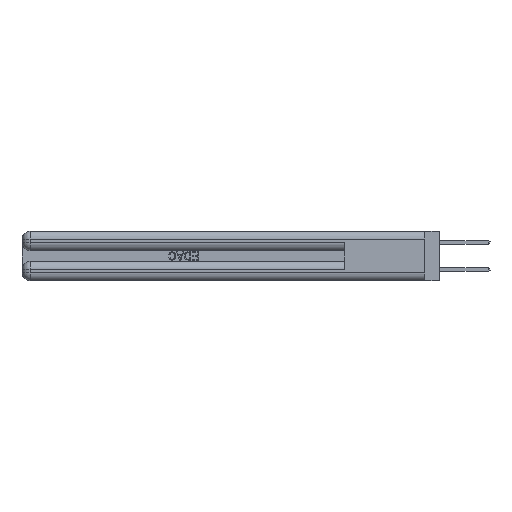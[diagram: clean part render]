
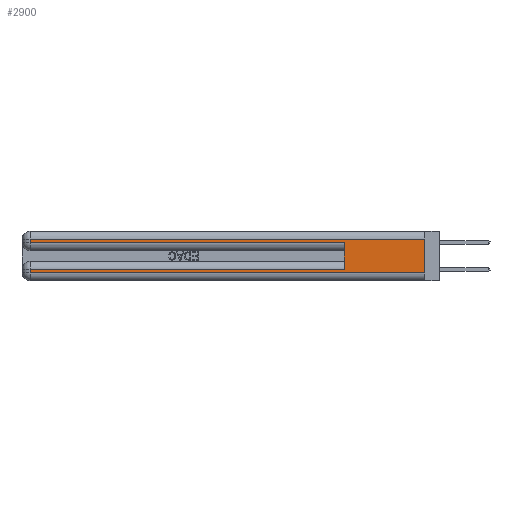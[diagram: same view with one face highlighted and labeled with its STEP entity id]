
A CAD part, left-side view. The second image highlights one B-rep face of the part: STEP entity #2900.
In plain terms, the highlighted planar face has unit normal (-1, 0, 0).
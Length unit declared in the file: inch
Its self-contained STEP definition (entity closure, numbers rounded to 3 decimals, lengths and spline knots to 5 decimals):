
#311 = VERTEX_POINT ( 'NONE', #35335 ) ;
#516 = ORIENTED_EDGE ( 'NONE', *, *, #13320, .F. ) ;
#2900 = ADVANCED_FACE ( 'NONE', ( #27308 ), #4148, .F. ) ;
#3091 = LINE ( 'NONE', #48751, #25488 ) ;
#3729 = DIRECTION ( 'NONE',  ( 0., 1., 0. ) ) ;
#3885 = EDGE_CURVE ( 'NONE', #311, #45356, #39031, .T. ) ;
#4148 = PLANE ( 'NONE',  #10611 ) ;
#4758 = CARTESIAN_POINT ( 'NONE',  ( 0., 0., 0.06 ) ) ;
#5013 = EDGE_CURVE ( 'NONE', #27637, #30637, #21609, .T. ) ;
#6375 = CARTESIAN_POINT ( 'NONE',  ( 0., 0.6, 0.285 ) ) ;
#6565 = ORIENTED_EDGE ( 'NONE', *, *, #25411, .T. ) ;
#8275 = DIRECTION ( 'NONE',  ( 0., 0., -1. ) ) ;
#8787 = LINE ( 'NONE', #36155, #49745 ) ;
#8927 = LINE ( 'NONE', #47568, #18885 ) ;
#9961 = ORIENTED_EDGE ( 'NONE', *, *, #5013, .T. ) ;
#10611 = AXIS2_PLACEMENT_3D ( 'NONE', #28104, #31907, #8275 ) ;
#11028 = VECTOR ( 'NONE', #49238, 39.37008 ) ;
#12165 = VERTEX_POINT ( 'NONE', #4758 ) ;
#12227 = VERTEX_POINT ( 'NONE', #31975 ) ;
#12584 = DIRECTION ( 'NONE',  ( 0., -1., 0. ) ) ;
#13320 = EDGE_CURVE ( 'NONE', #27637, #12165, #14397, .T. ) ;
#14397 = LINE ( 'NONE', #25874, #16201 ) ;
#16083 = VECTOR ( 'NONE', #33335, 39.37008 ) ;
#16201 = VECTOR ( 'NONE', #22701, 39.37008 ) ;
#16848 = DIRECTION ( 'NONE',  ( 0., 0., -1. ) ) ;
#17067 = VERTEX_POINT ( 'NONE', #25516 ) ;
#17086 = EDGE_CURVE ( 'NONE', #48255, #12165, #19767, .T. ) ;
#18885 = VECTOR ( 'NONE', #3729, 39.37008 ) ;
#19372 = CARTESIAN_POINT ( 'NONE',  ( 0., 0., 0.31 ) ) ;
#19767 = LINE ( 'NONE', #29303, #33404 ) ;
#21362 = EDGE_CURVE ( 'NONE', #17067, #45356, #8787, .T. ) ;
#21609 = LINE ( 'NONE', #47863, #11028 ) ;
#22701 = DIRECTION ( 'NONE',  ( 0., 0., -1. ) ) ;
#22913 = ORIENTED_EDGE ( 'NONE', *, *, #17086, .T. ) ;
#23932 = VECTOR ( 'NONE', #16848, 39.37008 ) ;
#24206 = ORIENTED_EDGE ( 'NONE', *, *, #21362, .T. ) ;
#25338 = ORIENTED_EDGE ( 'NONE', *, *, #3885, .F. ) ;
#25411 = EDGE_CURVE ( 'NONE', #30637, #17067, #3091, .T. ) ;
#25488 = VECTOR ( 'NONE', #44753, 39.37008 ) ;
#25516 = CARTESIAN_POINT ( 'NONE',  ( 0., 2.94, 0.285 ) ) ;
#25874 = CARTESIAN_POINT ( 'NONE',  ( 0., 0., 0.37 ) ) ;
#27308 = FACE_OUTER_BOUND ( 'NONE', #49842, .T. ) ;
#27637 = VERTEX_POINT ( 'NONE', #19372 ) ;
#27969 = CARTESIAN_POINT ( 'NONE',  ( 0., 2.94, 0.06 ) ) ;
#28104 = CARTESIAN_POINT ( 'NONE',  ( 0., 0., 0.37 ) ) ;
#29303 = CARTESIAN_POINT ( 'NONE',  ( 0., 0., 0.06 ) ) ;
#30637 = VERTEX_POINT ( 'NONE', #36204 ) ;
#31907 = DIRECTION ( 'NONE',  ( 1., 0., 0. ) ) ;
#31975 = CARTESIAN_POINT ( 'NONE',  ( 0., 2.94, 0.085 ) ) ;
#33274 = DIRECTION ( 'NONE',  ( 0., -1., 0. ) ) ;
#33335 = DIRECTION ( 'NONE',  ( 0., 0., 1. ) ) ;
#33404 = VECTOR ( 'NONE', #33274, 39.37008 ) ;
#33879 = EDGE_CURVE ( 'NONE', #12227, #48255, #43159, .T. ) ;
#35335 = CARTESIAN_POINT ( 'NONE',  ( 0., 0.6, 0.085 ) ) ;
#36155 = CARTESIAN_POINT ( 'NONE',  ( 0., 0., 0.285 ) ) ;
#36204 = CARTESIAN_POINT ( 'NONE',  ( 0., 2.94, 0.31 ) ) ;
#38489 = ORIENTED_EDGE ( 'NONE', *, *, #43011, .T. ) ;
#39031 = LINE ( 'NONE', #49585, #16083 ) ;
#43011 = EDGE_CURVE ( 'NONE', #311, #12227, #8927, .T. ) ;
#43159 = LINE ( 'NONE', #48215, #23932 ) ;
#44753 = DIRECTION ( 'NONE',  ( 0., 0., -1. ) ) ;
#45356 = VERTEX_POINT ( 'NONE', #6375 ) ;
#47568 = CARTESIAN_POINT ( 'NONE',  ( 0., 0., 0.085 ) ) ;
#47863 = CARTESIAN_POINT ( 'NONE',  ( 0., 0., 0.31 ) ) ;
#48215 = CARTESIAN_POINT ( 'NONE',  ( 0., 2.94, 0.37 ) ) ;
#48255 = VERTEX_POINT ( 'NONE', #27969 ) ;
#48751 = CARTESIAN_POINT ( 'NONE',  ( 0., 2.94, 0.37 ) ) ;
#49238 = DIRECTION ( 'NONE',  ( 0., 1., 0. ) ) ;
#49585 = CARTESIAN_POINT ( 'NONE',  ( 0., 0.6, 0.145 ) ) ;
#49745 = VECTOR ( 'NONE', #12584, 39.37008 ) ;
#49842 = EDGE_LOOP ( 'NONE', ( #516, #9961, #6565, #24206, #25338, #38489, #49868, #22913 ) ) ;
#49868 = ORIENTED_EDGE ( 'NONE', *, *, #33879, .T. ) ;
